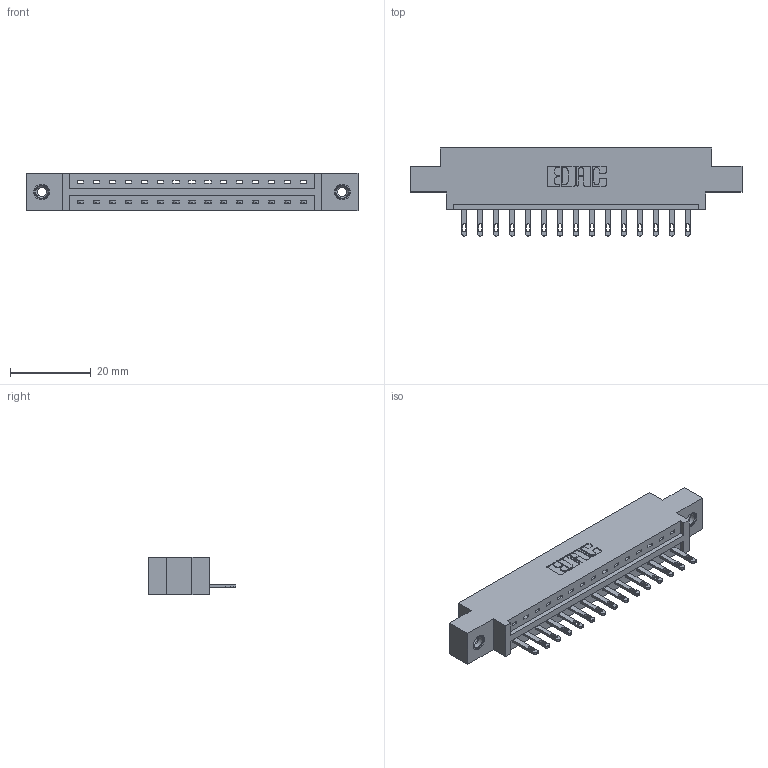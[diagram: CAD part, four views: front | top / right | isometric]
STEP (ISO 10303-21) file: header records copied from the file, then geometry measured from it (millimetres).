
FILE_DESCRIPTION (( 'STEP AP203' ), '1' );
FILE_NAME ('887-015-500-608.STEP', '2020-09-20T17:05:57', ( '' ), ( '' ), 'SwSTEP 2.0', 'SolidWorks 2020', '' );
FILE_SCHEMA (( 'CONFIG_CONTROL_DESIGN' ));
Length unit declared in the file: inch
Products named in the file (4): 887-015-500-608; 345-292-001_345-293-100; 345-250-001_345-250-003-102; 837 Part_0.170 Offset - 0.156 Dia-TI
Assembly tree (18 placements, depth 2):
  887-015-500-608
    837 Part_0.170 Offset - 0.156 Dia-TI
    345-292-001_345-293-100  x15
    345-250-001_345-250-003-102  x2
Bounding box: 82.45 x 21.85 x 9.4 mm (x, y, z)
Volume: 8116.5 mm3; surface area: 8398.5 mm2
Topology: 18 solids, 18 shells, 1048 faces, 3159 edges, 2098 vertices
Faces by surface type: plane 706, cylinder 326, cone 12, torus 4
Entity records: 15890 total; most frequent: CARTESIAN_POINT 2746, ORIENTED_EDGE 2690, DIRECTION 2401, EDGE_CURVE 1345, VECTOR 1193, LINE 1193, VERTEX_POINT 892, AXIS2_PLACEMENT_3D 604
